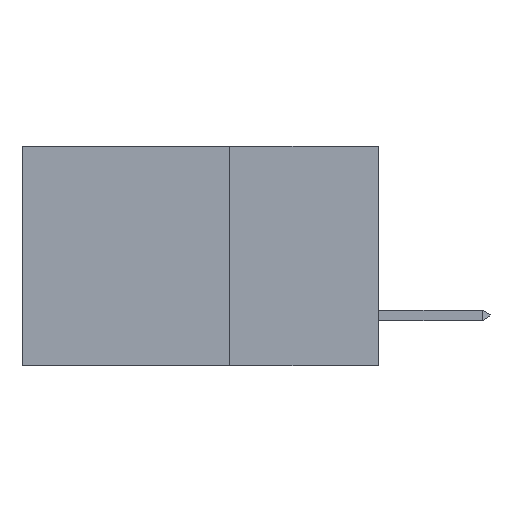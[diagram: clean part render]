
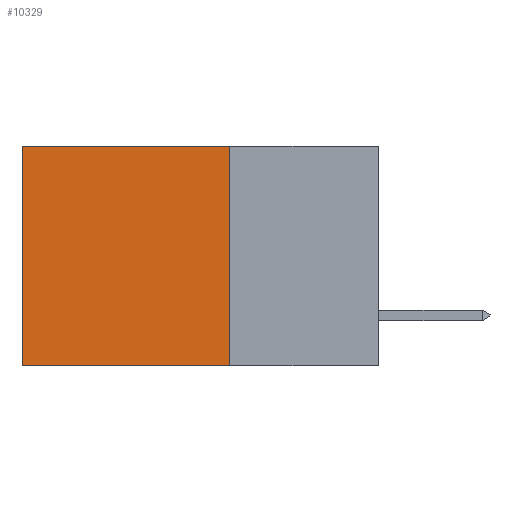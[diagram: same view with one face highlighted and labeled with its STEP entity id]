
A CAD part, left-side view. The second image highlights one B-rep face of the part: STEP entity #10329.
In plain terms, the highlighted planar face has unit normal (-1, 0, 0).
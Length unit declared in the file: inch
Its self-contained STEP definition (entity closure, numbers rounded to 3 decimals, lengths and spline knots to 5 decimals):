
#100 = DIRECTION ( 'NONE',  ( 1., 0., 0. ) ) ;
#125 = VERTEX_POINT ( 'NONE', #6962 ) ;
#727 = VECTOR ( 'NONE', #3612, 39.37008 ) ;
#965 = AXIS2_PLACEMENT_3D ( 'NONE', #9924, #100, #7972 ) ;
#1332 = LINE ( 'NONE', #5517, #6616 ) ;
#1562 = DIRECTION ( 'NONE',  ( 0., 0., -1. ) ) ;
#1597 = ORIENTED_EDGE ( 'NONE', *, *, #10726, .F. ) ;
#1693 = DIRECTION ( 'NONE',  ( 0., 1., 0. ) ) ;
#2062 = VERTEX_POINT ( 'NONE', #5003 ) ;
#2168 = VERTEX_POINT ( 'NONE', #10782 ) ;
#2233 = ORIENTED_EDGE ( 'NONE', *, *, #6729, .F. ) ;
#2428 = LINE ( 'NONE', #5929, #3072 ) ;
#2553 = ORIENTED_EDGE ( 'NONE', *, *, #3391, .T. ) ;
#2828 = FACE_OUTER_BOUND ( 'NONE', #7437, .T. ) ;
#3072 = VECTOR ( 'NONE', #1562, 39.37008 ) ;
#3391 = EDGE_CURVE ( 'NONE', #2168, #125, #6921, .T. ) ;
#3612 = DIRECTION ( 'NONE',  ( 0., 0., -1. ) ) ;
#4531 = CARTESIAN_POINT ( 'NONE',  ( 0.2615, 0.25, -0.37 ) ) ;
#5003 = CARTESIAN_POINT ( 'NONE',  ( 0.2615, 0.25, -0.37 ) ) ;
#5517 = CARTESIAN_POINT ( 'NONE',  ( 0.2615, 0.25, -0.37 ) ) ;
#5650 = EDGE_CURVE ( 'NONE', #125, #9695, #2428, .T. ) ;
#5929 = CARTESIAN_POINT ( 'NONE',  ( 0.2615, 0.6, -0.37 ) ) ;
#6616 = VECTOR ( 'NONE', #10068, 39.37008 ) ;
#6729 = EDGE_CURVE ( 'NONE', #2062, #9695, #1332, .T. ) ;
#6820 = ORIENTED_EDGE ( 'NONE', *, *, #5650, .T. ) ;
#6921 = LINE ( 'NONE', #10432, #9401 ) ;
#6962 = CARTESIAN_POINT ( 'NONE',  ( 0.2615, 0.6, 0. ) ) ;
#7437 = EDGE_LOOP ( 'NONE', ( #6820, #2233, #1597, #2553 ) ) ;
#7972 = DIRECTION ( 'NONE',  ( 0., 0., -1. ) ) ;
#8008 = LINE ( 'NONE', #4531, #727 ) ;
#8622 = CARTESIAN_POINT ( 'NONE',  ( 0.2615, 0.6, -0.37 ) ) ;
#9401 = VECTOR ( 'NONE', #1693, 39.37008 ) ;
#9695 = VERTEX_POINT ( 'NONE', #8622 ) ;
#9924 = CARTESIAN_POINT ( 'NONE',  ( 0.2615, 0.25, -0.37 ) ) ;
#9977 = PLANE ( 'NONE',  #965 ) ;
#10068 = DIRECTION ( 'NONE',  ( 0., 1., 0. ) ) ;
#10329 = ADVANCED_FACE ( 'NONE', ( #2828 ), #9977, .F. ) ;
#10432 = CARTESIAN_POINT ( 'NONE',  ( 0.2615, 0.25, 0. ) ) ;
#10726 = EDGE_CURVE ( 'NONE', #2168, #2062, #8008, .T. ) ;
#10782 = CARTESIAN_POINT ( 'NONE',  ( 0.2615, 0.25, 0. ) ) ;
